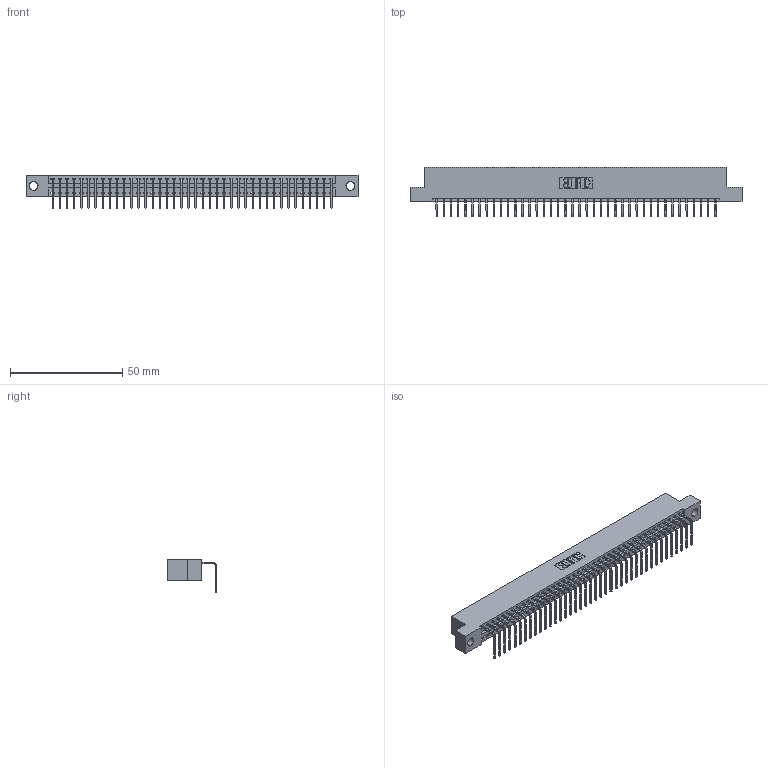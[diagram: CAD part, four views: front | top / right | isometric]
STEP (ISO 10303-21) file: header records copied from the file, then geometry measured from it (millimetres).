
FILE_DESCRIPTION (( 'STEP AP203' ), '1' );
FILE_NAME ('346-040-558-104.STEP', '2022-05-07T10:14:49', ( '' ), ( '' ), 'SwSTEP 2.0', 'SolidWorks 2020', '' );
FILE_SCHEMA (( 'CONFIG_CONTROL_DESIGN' ));
Length unit declared in the file: inch
Products named in the file (3): 345-292-001_558 Tail - 2; 346-040-558-104; 346 Part_Flush Mounting Lugs - 0.156 Dia-TH
Assembly tree (41 placements, depth 2):
  346-040-558-104
    346 Part_Flush Mounting Lugs - 0.156 Dia-TH
    345-292-001_558 Tail - 2  x40
Bounding box: 147.57 x 22.16 x 14.73 mm (x, y, z)
Volume: 14139.6 mm3; surface area: 18283.5 mm2
Topology: 41 solids, 41 shells, 2536 faces, 7645 edges, 5042 vertices
Faces by surface type: plane 1770, cylinder 766
Entity records: 25597 total; most frequent: CARTESIAN_POINT 4398, ORIENTED_EDGE 4370, DIRECTION 3881, EDGE_CURVE 2185, VECTOR 1893, LINE 1893, VERTEX_POINT 1454, AXIS2_PLACEMENT_3D 994
